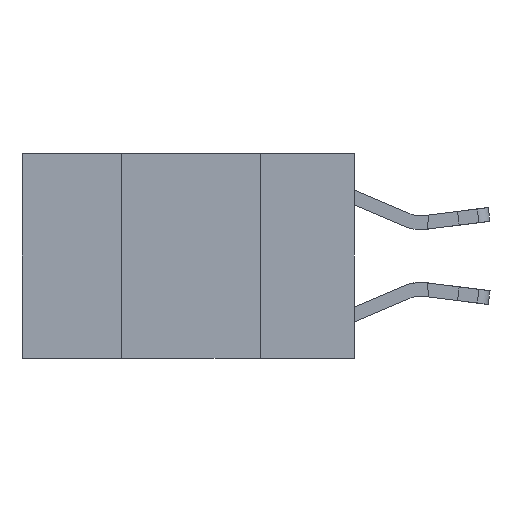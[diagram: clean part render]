
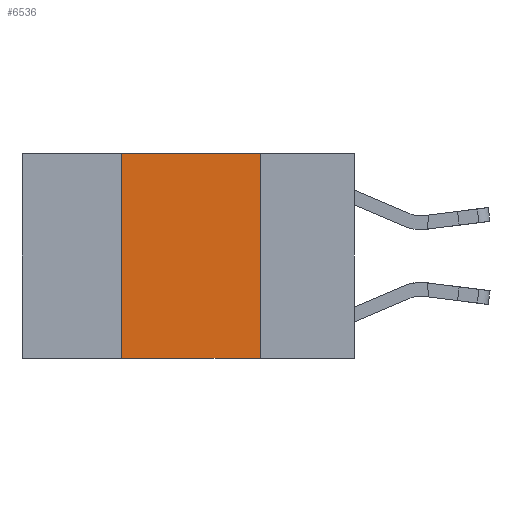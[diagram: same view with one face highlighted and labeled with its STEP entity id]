
A CAD part, left-side view. The second image highlights one B-rep face of the part: STEP entity #6536.
In plain terms, the highlighted planar face has unit normal (-1, 0, 0).
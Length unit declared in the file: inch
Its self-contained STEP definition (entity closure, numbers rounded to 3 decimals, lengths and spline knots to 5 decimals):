
#1717 = ORIENTED_EDGE ( 'NONE', *, *, #17090, .T. ) ;
#1764 = VECTOR ( 'NONE', #8231, 39.37008 ) ;
#2033 = EDGE_LOOP ( 'NONE', ( #18882, #9057, #18105, #1717 ) ) ;
#2554 = VERTEX_POINT ( 'NONE', #19940 ) ;
#2824 = VECTOR ( 'NONE', #14933, 39.37008 ) ;
#3430 = LINE ( 'NONE', #14756, #1764 ) ;
#4010 = VERTEX_POINT ( 'NONE', #10405 ) ;
#4873 = LINE ( 'NONE', #11223, #17369 ) ;
#4887 = AXIS2_PLACEMENT_3D ( 'NONE', #7045, #16396, #6836 ) ;
#5578 = EDGE_CURVE ( 'NONE', #2554, #18748, #19833, .T. ) ;
#6102 = EDGE_CURVE ( 'NONE', #19278, #2554, #3430, .T. ) ;
#6536 = ADVANCED_FACE ( 'NONE', ( #14735 ), #7247, .F. ) ;
#6836 = DIRECTION ( 'NONE',  ( 0., 0., -1. ) ) ;
#7045 = CARTESIAN_POINT ( 'NONE',  ( 0., 0.6, 0. ) ) ;
#7247 = PLANE ( 'NONE',  #4887 ) ;
#8231 = DIRECTION ( 'NONE',  ( 0., -1., 0. ) ) ;
#8514 = CARTESIAN_POINT ( 'NONE',  ( 0., 0.17, 0. ) ) ;
#9057 = ORIENTED_EDGE ( 'NONE', *, *, #6102, .F. ) ;
#10405 = CARTESIAN_POINT ( 'NONE',  ( 0., 0.42, -0.37 ) ) ;
#10700 = DIRECTION ( 'NONE',  ( 0., 0., 1. ) ) ;
#10705 = CARTESIAN_POINT ( 'NONE',  ( 0., 0.17, -0.37 ) ) ;
#10799 = CARTESIAN_POINT ( 'NONE',  ( 0., 0.42, 0. ) ) ;
#11223 = CARTESIAN_POINT ( 'NONE',  ( 0., 0.6, -0.37 ) ) ;
#12050 = LINE ( 'NONE', #10799, #20320 ) ;
#12691 = EDGE_CURVE ( 'NONE', #4010, #19278, #12050, .T. ) ;
#14735 = FACE_OUTER_BOUND ( 'NONE', #2033, .T. ) ;
#14756 = CARTESIAN_POINT ( 'NONE',  ( 0., 0.6, 0. ) ) ;
#14933 = DIRECTION ( 'NONE',  ( 0., 0., -1. ) ) ;
#16396 = DIRECTION ( 'NONE',  ( 1., 0., 0. ) ) ;
#17090 = EDGE_CURVE ( 'NONE', #4010, #18748, #4873, .T. ) ;
#17369 = VECTOR ( 'NONE', #17569, 39.37008 ) ;
#17569 = DIRECTION ( 'NONE',  ( 0., -1., 0. ) ) ;
#18105 = ORIENTED_EDGE ( 'NONE', *, *, #12691, .F. ) ;
#18748 = VERTEX_POINT ( 'NONE', #10705 ) ;
#18882 = ORIENTED_EDGE ( 'NONE', *, *, #5578, .F. ) ;
#19278 = VERTEX_POINT ( 'NONE', #20359 ) ;
#19833 = LINE ( 'NONE', #8514, #2824 ) ;
#19940 = CARTESIAN_POINT ( 'NONE',  ( 0., 0.17, 0. ) ) ;
#20320 = VECTOR ( 'NONE', #10700, 39.37008 ) ;
#20359 = CARTESIAN_POINT ( 'NONE',  ( 0., 0.42, 0. ) ) ;
